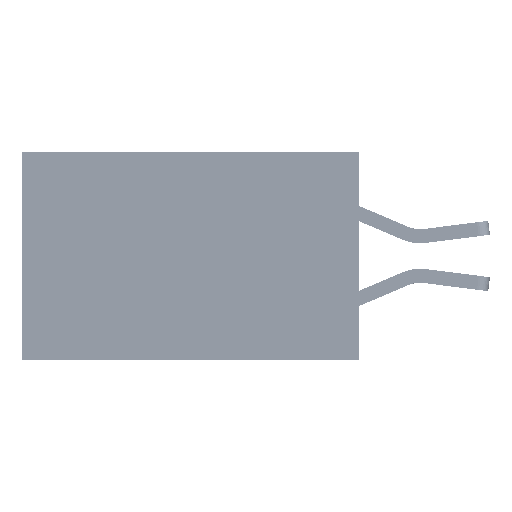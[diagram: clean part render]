
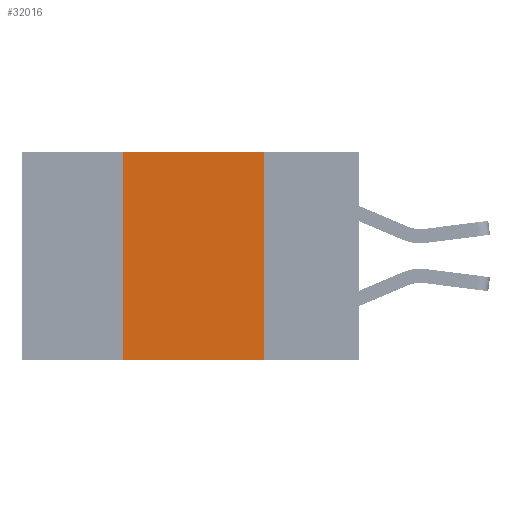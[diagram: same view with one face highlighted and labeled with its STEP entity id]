
A CAD part, left-side view. The second image highlights one B-rep face of the part: STEP entity #32016.
In plain terms, the highlighted planar face has unit normal (-1, 0, 0).
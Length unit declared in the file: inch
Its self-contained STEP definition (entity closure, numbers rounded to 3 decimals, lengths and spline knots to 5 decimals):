
#1365 = EDGE_CURVE ( 'NONE', #27743, #32127, #3645, .T. ) ;
#3645 = LINE ( 'NONE', #44829, #47396 ) ;
#3935 = ORIENTED_EDGE ( 'NONE', *, *, #9523, .F. ) ;
#5610 = DIRECTION ( 'NONE',  ( 0., -1., 0. ) ) ;
#5848 = CARTESIAN_POINT ( 'NONE',  ( 0., 0.17, 0. ) ) ;
#7304 = ORIENTED_EDGE ( 'NONE', *, *, #1365, .T. ) ;
#7588 = VECTOR ( 'NONE', #39198, 39.37008 ) ;
#8565 = ORIENTED_EDGE ( 'NONE', *, *, #40054, .F. ) ;
#9523 = EDGE_CURVE ( 'NONE', #27743, #47823, #35222, .T. ) ;
#9728 = CARTESIAN_POINT ( 'NONE',  ( 0., 0.17, 0. ) ) ;
#11176 = AXIS2_PLACEMENT_3D ( 'NONE', #17494, #43570, #21634 ) ;
#11207 = DIRECTION ( 'NONE',  ( 0., -1., 0. ) ) ;
#11307 = EDGE_LOOP ( 'NONE', ( #32249, #8565, #3935, #7304 ) ) ;
#15314 = EDGE_CURVE ( 'NONE', #29586, #32127, #47725, .T. ) ;
#16122 = LINE ( 'NONE', #42659, #17799 ) ;
#16251 = DIRECTION ( 'NONE',  ( 0., 0., 1. ) ) ;
#17494 = CARTESIAN_POINT ( 'NONE',  ( 0., 0.6, 0. ) ) ;
#17799 = VECTOR ( 'NONE', #5610, 39.37008 ) ;
#20918 = FACE_OUTER_BOUND ( 'NONE', #11307, .T. ) ;
#21634 = DIRECTION ( 'NONE',  ( 0., 0., -1. ) ) ;
#27743 = VERTEX_POINT ( 'NONE', #27787 ) ;
#27787 = CARTESIAN_POINT ( 'NONE',  ( 0., 0.42, -0.37 ) ) ;
#29586 = VERTEX_POINT ( 'NONE', #5848 ) ;
#32016 = ADVANCED_FACE ( 'NONE', ( #20918 ), #39900, .F. ) ;
#32127 = VERTEX_POINT ( 'NONE', #33558 ) ;
#32249 = ORIENTED_EDGE ( 'NONE', *, *, #15314, .F. ) ;
#33558 = CARTESIAN_POINT ( 'NONE',  ( 0., 0.17, -0.37 ) ) ;
#35222 = LINE ( 'NONE', #46451, #41521 ) ;
#35615 = CARTESIAN_POINT ( 'NONE',  ( 0., 0.42, 0. ) ) ;
#39198 = DIRECTION ( 'NONE',  ( 0., 0., -1. ) ) ;
#39900 = PLANE ( 'NONE',  #11176 ) ;
#40054 = EDGE_CURVE ( 'NONE', #47823, #29586, #16122, .T. ) ;
#41521 = VECTOR ( 'NONE', #16251, 39.37008 ) ;
#42659 = CARTESIAN_POINT ( 'NONE',  ( 0., 0.6, 0. ) ) ;
#43570 = DIRECTION ( 'NONE',  ( 1., 0., 0. ) ) ;
#44829 = CARTESIAN_POINT ( 'NONE',  ( 0., 0.6, -0.37 ) ) ;
#46451 = CARTESIAN_POINT ( 'NONE',  ( 0., 0.42, 0. ) ) ;
#47396 = VECTOR ( 'NONE', #11207, 39.37008 ) ;
#47725 = LINE ( 'NONE', #9728, #7588 ) ;
#47823 = VERTEX_POINT ( 'NONE', #35615 ) ;
